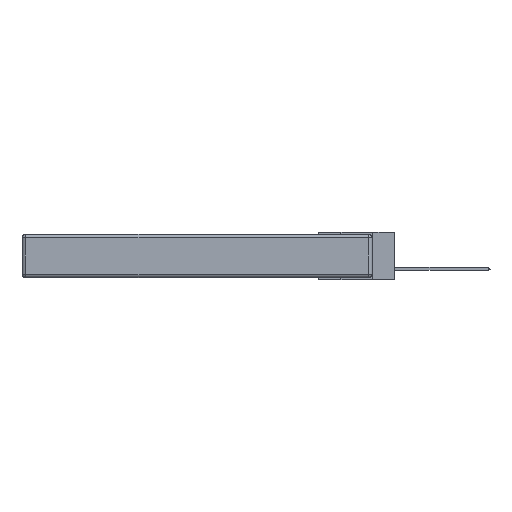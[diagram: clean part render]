
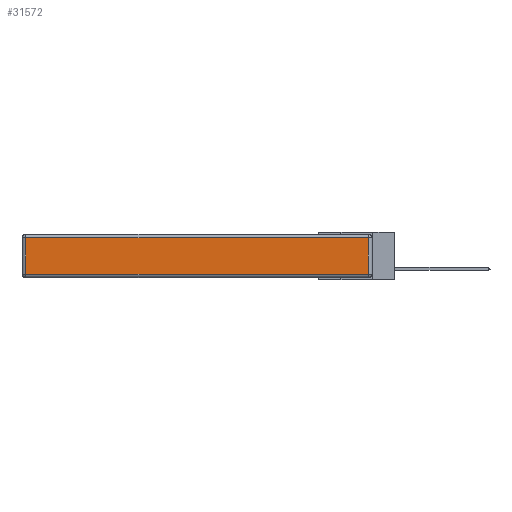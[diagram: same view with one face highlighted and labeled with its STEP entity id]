
A CAD part, left-side view. The second image highlights one B-rep face of the part: STEP entity #31572.
In plain terms, the highlighted planar face has unit normal (-1, 0, 0).
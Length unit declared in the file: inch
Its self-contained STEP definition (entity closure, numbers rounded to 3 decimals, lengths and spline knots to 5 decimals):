
#1456 = CARTESIAN_POINT ( 'NONE',  ( 0., 2.72, -0.313 ) ) ;
#4529 = EDGE_CURVE ( 'NONE', #31870, #21207, #26165, .T. ) ;
#4653 = PLANE ( 'NONE',  #5338 ) ;
#4840 = CARTESIAN_POINT ( 'NONE',  ( 0., 2.75, -0.03 ) ) ;
#4963 = CARTESIAN_POINT ( 'NONE',  ( 0., 0.03, -0.343 ) ) ;
#5338 = AXIS2_PLACEMENT_3D ( 'NONE', #22516, #28023, #30655 ) ;
#7765 = EDGE_LOOP ( 'NONE', ( #32121, #18367, #12359, #29015 ) ) ;
#9583 = FACE_OUTER_BOUND ( 'NONE', #7765, .T. ) ;
#11269 = CARTESIAN_POINT ( 'NONE',  ( 0., 0., -0.313 ) ) ;
#12027 = VECTOR ( 'NONE', #16291, 39.37008 ) ;
#12359 = ORIENTED_EDGE ( 'NONE', *, *, #25830, .T. ) ;
#12483 = CARTESIAN_POINT ( 'NONE',  ( 0., 2.72, -0.343 ) ) ;
#14470 = LINE ( 'NONE', #11269, #12027 ) ;
#14760 = LINE ( 'NONE', #12483, #23598 ) ;
#16291 = DIRECTION ( 'NONE',  ( 0., -1., 0. ) ) ;
#16570 = LINE ( 'NONE', #4840, #29461 ) ;
#18367 = ORIENTED_EDGE ( 'NONE', *, *, #4529, .T. ) ;
#18554 = VECTOR ( 'NONE', #26052, 39.37008 ) ;
#19164 = CARTESIAN_POINT ( 'NONE',  ( 0., 2.72, -0.03 ) ) ;
#19697 = EDGE_CURVE ( 'NONE', #26492, #31870, #14470, .T. ) ;
#21207 = VERTEX_POINT ( 'NONE', #28716 ) ;
#22516 = CARTESIAN_POINT ( 'NONE',  ( 0., 0., -0.343 ) ) ;
#22579 = DIRECTION ( 'NONE',  ( 0., 1., 0. ) ) ;
#23598 = VECTOR ( 'NONE', #33175, 39.37008 ) ;
#25830 = EDGE_CURVE ( 'NONE', #21207, #31400, #16570, .T. ) ;
#26052 = DIRECTION ( 'NONE',  ( 0., 0., 1. ) ) ;
#26165 = LINE ( 'NONE', #4963, #18554 ) ;
#26492 = VERTEX_POINT ( 'NONE', #1456 ) ;
#27629 = CARTESIAN_POINT ( 'NONE',  ( 0., 0.03, -0.313 ) ) ;
#28023 = DIRECTION ( 'NONE',  ( -1., 0., 0. ) ) ;
#28716 = CARTESIAN_POINT ( 'NONE',  ( 0., 0.03, -0.03 ) ) ;
#29015 = ORIENTED_EDGE ( 'NONE', *, *, #33039, .T. ) ;
#29461 = VECTOR ( 'NONE', #22579, 39.37008 ) ;
#30655 = DIRECTION ( 'NONE',  ( 0., 0., 1. ) ) ;
#31400 = VERTEX_POINT ( 'NONE', #19164 ) ;
#31572 = ADVANCED_FACE ( 'NONE', ( #9583 ), #4653, .T. ) ;
#31870 = VERTEX_POINT ( 'NONE', #27629 ) ;
#32121 = ORIENTED_EDGE ( 'NONE', *, *, #19697, .T. ) ;
#33039 = EDGE_CURVE ( 'NONE', #31400, #26492, #14760, .T. ) ;
#33175 = DIRECTION ( 'NONE',  ( 0., 0., -1. ) ) ;
